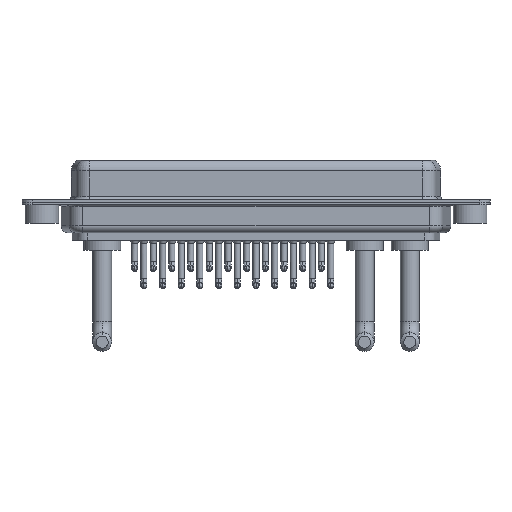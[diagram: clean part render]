
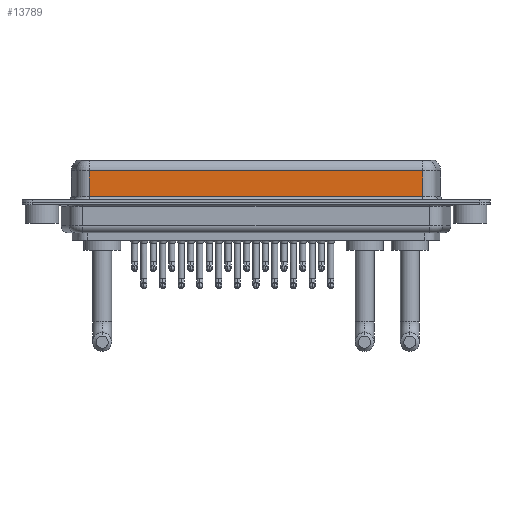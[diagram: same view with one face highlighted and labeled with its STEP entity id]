
A CAD part, front view. The second image highlights one B-rep face of the part: STEP entity #13789.
In plain terms, the highlighted planar face has unit normal (0, -1, 0).
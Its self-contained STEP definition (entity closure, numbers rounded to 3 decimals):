
#373 = VERTEX_POINT ( 'NONE', #5315 ) ;
#1070 = PLANE ( 'NONE',  #17197 ) ;
#1284 = CARTESIAN_POINT ( 'NONE',  ( 56.462, -3.95, 0.9 ) ) ;
#2669 = EDGE_CURVE ( 'NONE', #373, #9989, #2856, .T. ) ;
#2856 = LINE ( 'NONE', #6345, #3011 ) ;
#3011 = VECTOR ( 'NONE', #17145, 1000. ) ;
#3123 = DIRECTION ( 'NONE',  ( -1., 0., 0. ) ) ;
#4822 = LINE ( 'NONE', #6979, #21197 ) ;
#4838 = CARTESIAN_POINT ( 'NONE',  ( 56.462, -3.95, 0.9 ) ) ;
#5315 = CARTESIAN_POINT ( 'NONE',  ( 7.038, -3.95, 4.65 ) ) ;
#5380 = CARTESIAN_POINT ( 'NONE',  ( 56.462, -3.95, 6.4 ) ) ;
#5744 = LINE ( 'NONE', #5380, #10505 ) ;
#5956 = EDGE_LOOP ( 'NONE', ( #12728, #17968, #6988, #14229 ) ) ;
#6345 = CARTESIAN_POINT ( 'NONE',  ( 7.038, -3.95, 6.4 ) ) ;
#6739 = DIRECTION ( 'NONE',  ( 0., 0., 1. ) ) ;
#6979 = CARTESIAN_POINT ( 'NONE',  ( 56.462, -3.95, 4.65 ) ) ;
#6988 = ORIENTED_EDGE ( 'NONE', *, *, #2669, .T. ) ;
#8711 = EDGE_CURVE ( 'NONE', #10403, #373, #4822, .T. ) ;
#9748 = EDGE_CURVE ( 'NONE', #10403, #13279, #5744, .T. ) ;
#9989 = VERTEX_POINT ( 'NONE', #21460 ) ;
#10403 = VERTEX_POINT ( 'NONE', #20481 ) ;
#10409 = DIRECTION ( 'NONE',  ( 1., 0., 0. ) ) ;
#10505 = VECTOR ( 'NONE', #14983, 1000. ) ;
#10565 = VECTOR ( 'NONE', #10409, 1000. ) ;
#12728 = ORIENTED_EDGE ( 'NONE', *, *, #9748, .F. ) ;
#13279 = VERTEX_POINT ( 'NONE', #4838 ) ;
#13789 = ADVANCED_FACE ( 'NONE', ( #14186 ), #1070, .F. ) ;
#14186 = FACE_OUTER_BOUND ( 'NONE', #5956, .T. ) ;
#14229 = ORIENTED_EDGE ( 'NONE', *, *, #21931, .T. ) ;
#14983 = DIRECTION ( 'NONE',  ( 0., 0., -1. ) ) ;
#17145 = DIRECTION ( 'NONE',  ( 0., 0., -1. ) ) ;
#17197 = AXIS2_PLACEMENT_3D ( 'NONE', #21509, #17656, #6739 ) ;
#17254 = LINE ( 'NONE', #1284, #10565 ) ;
#17656 = DIRECTION ( 'NONE',  ( 0., 1., 0. ) ) ;
#17968 = ORIENTED_EDGE ( 'NONE', *, *, #8711, .T. ) ;
#20481 = CARTESIAN_POINT ( 'NONE',  ( 56.462, -3.95, 4.65 ) ) ;
#21197 = VECTOR ( 'NONE', #3123, 1000. ) ;
#21460 = CARTESIAN_POINT ( 'NONE',  ( 7.038, -3.95, 0.9 ) ) ;
#21509 = CARTESIAN_POINT ( 'NONE',  ( 56.462, -3.95, 6.4 ) ) ;
#21931 = EDGE_CURVE ( 'NONE', #9989, #13279, #17254, .T. ) ;
